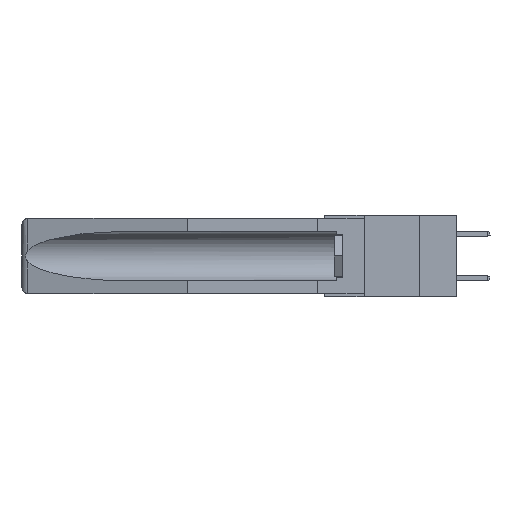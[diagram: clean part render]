
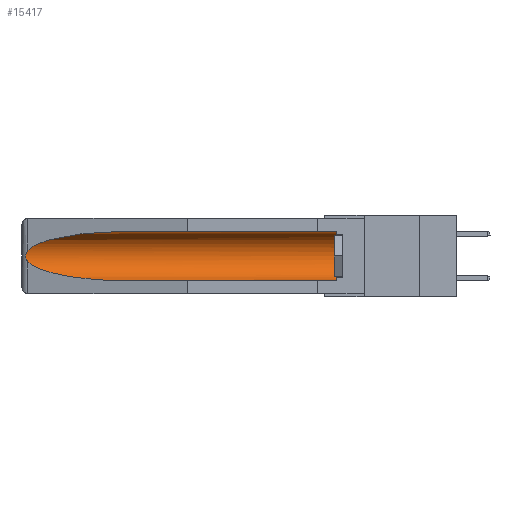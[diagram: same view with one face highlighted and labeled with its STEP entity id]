
A CAD part, left-side view. The second image highlights one B-rep face of the part: STEP entity #15417.
In plain terms, the highlighted cylindrical face has radius 2.857 mm (diameter 5.715 mm), a partial arc.
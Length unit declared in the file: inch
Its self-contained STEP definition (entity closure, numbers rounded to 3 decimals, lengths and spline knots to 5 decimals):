
#425 = CYLINDRICAL_SURFACE ( 'NONE', #18403, 0.1125 ) ;
#969 = ORIENTED_EDGE ( 'NONE', *, *, #23321, .T. ) ;
#1375 = CARTESIAN_POINT ( 'NONE',  ( 0.155, 1.07973, -0.059 ) ) ;
#1829 = CARTESIAN_POINT ( 'NONE',  ( 0.2675, 1.53308, -0.17534 ) ) ;
#2647 = CARTESIAN_POINT ( 'NONE',  ( 0.155, -0.30754, -0.284 ) ) ;
#3432 = DIRECTION ( 'NONE',  ( 0., -1., 0. ) ) ;
#3469 = CARTESIAN_POINT ( 'NONE',  ( 0.155, 1.07973, -0.059 ) ) ;
#3788 = CARTESIAN_POINT ( 'NONE',  ( 0.21114, 1.30732, -0.284 ) ) ;
#3941 = FACE_OUTER_BOUND ( 'NONE', #4573, .T. ) ;
#4108 = ORIENTED_EDGE ( 'NONE', *, *, #27617, .T. ) ;
#4573 = EDGE_LOOP ( 'NONE', ( #5721, #26102, #969, #15722, #8129, #4108 ) ) ;
#4890 = DIRECTION ( 'NONE',  ( 0., 1., 0. ) ) ;
#5669 = CARTESIAN_POINT ( 'NONE',  ( 0.155, -0.30754, -0.059 ) ) ;
#5721 = ORIENTED_EDGE ( 'NONE', *, *, #13810, .T. ) ;
#6030 = CARTESIAN_POINT ( 'NONE',  ( 0.25451, 1.48313, -0.24835 ) ) ;
#6208 = CARTESIAN_POINT ( 'NONE',  ( 0.2673, 1.5327, -0.16383 ) ) ;
#6499 = CARTESIAN_POINT ( 'NONE',  ( 0.2673, 1.53269, -0.17917 ) ) ;
#6960 = CIRCLE ( 'NONE', #20569, 0.1125 ) ;
#8078 = B_SPLINE_CURVE_WITH_KNOTS ( 'NONE', 3,
 ( #19342, #12297, #22026, #6208, #23766, #1829, #6499, #26342, #15083, #15363 ),
 .UNSPECIFIED., .F., .F.,
 ( 4, 2, 2, 2, 4 ),
 ( 0., 0.00029, 0.00058, 0.00087, 0.00117 ),
 .UNSPECIFIED. ) ;
#8129 = ORIENTED_EDGE ( 'NONE', *, *, #27659, .T. ) ;
#8328 = CARTESIAN_POINT ( 'NONE',  ( 0.155, 1.07973, -0.284 ) ) ;
#8351 = CARTESIAN_POINT ( 'NONE',  ( 0.25451, 1.48313, -0.09465 ) ) ;
#9335 = VERTEX_POINT ( 'NONE', #19766 ) ;
#9618 = DIRECTION ( 'NONE',  ( 0., 0., 1. ) ) ;
#11396 = VERTEX_POINT ( 'NONE', #3469 ) ;
#12297 = CARTESIAN_POINT ( 'NONE',  ( 0.26597, 1.52961, -0.15275 ) ) ;
#13810 = EDGE_CURVE ( 'NONE', #11396, #9335, #17532, .T. ) ;
#14111 = CARTESIAN_POINT ( 'NONE',  ( 0.155, -0.30754, -0.1715 ) ) ;
#15083 = CARTESIAN_POINT ( 'NONE',  ( 0.26597, 1.5296, -0.19026 ) ) ;
#15363 = CARTESIAN_POINT ( 'NONE',  ( 0.26537, 1.52718, -0.19328 ) ) ;
#15389 = VERTEX_POINT ( 'NONE', #16059 ) ;
#15417 = ADVANCED_FACE ( 'NONE', ( #3941 ), #425, .F. ) ;
#15722 = ORIENTED_EDGE ( 'NONE', *, *, #21259, .F. ) ;
#16059 = CARTESIAN_POINT ( 'NONE',  ( 0.155, 0.126, -0.059 ) ) ;
#16081 = CARTESIAN_POINT ( 'NONE',  ( 0.26537, 1.52718, -0.19328 ) ) ;
#16773 = CARTESIAN_POINT ( 'NONE',  ( 0.155, 0.126, -0.1715 ) ) ;
#17495 = CARTESIAN_POINT ( 'NONE',  ( 0.155, 1.07973, -0.284 ) ) ;
#17532 =( BOUNDED_CURVE ( )  B_SPLINE_CURVE ( 3, ( #1375, #21564, #8351, #28022 ),
 .UNSPECIFIED., .F., .F. ) 
 B_SPLINE_CURVE_WITH_KNOTS ( ( 4, 4 ),
 ( 4.71239, 6.08839 ),
 .UNSPECIFIED. ) 
 CURVE ( )  GEOMETRIC_REPRESENTATION_ITEM ( )  RATIONAL_B_SPLINE_CURVE ( ( 1., 0.848, 0.848, 1. ) ) 
 REPRESENTATION_ITEM ( '' )  );
#17902 = VERTEX_POINT ( 'NONE', #17495 ) ;
#18403 = AXIS2_PLACEMENT_3D ( 'NONE', #14111, #27607, #9618 ) ;
#19000 = DIRECTION ( 'NONE',  ( 0., 0., 1. ) ) ;
#19342 = CARTESIAN_POINT ( 'NONE',  ( 0.26537, 1.52718, -0.14972 ) ) ;
#19766 = CARTESIAN_POINT ( 'NONE',  ( 0.26537, 1.52718, -0.14972 ) ) ;
#20569 = AXIS2_PLACEMENT_3D ( 'NONE', #16773, #3432, #19000 ) ;
#20697 = VERTEX_POINT ( 'NONE', #22588 ) ;
#21259 = EDGE_CURVE ( 'NONE', #20697, #17902, #24244, .T. ) ;
#21494 = EDGE_CURVE ( 'NONE', #9335, #22833, #8078, .T. ) ;
#21564 = CARTESIAN_POINT ( 'NONE',  ( 0.21114, 1.30732, -0.059 ) ) ;
#22026 = CARTESIAN_POINT ( 'NONE',  ( 0.26654, 1.53092, -0.15636 ) ) ;
#22588 = CARTESIAN_POINT ( 'NONE',  ( 0.155, 0.126, -0.284 ) ) ;
#22833 = VERTEX_POINT ( 'NONE', #16081 ) ;
#23321 = EDGE_CURVE ( 'NONE', #22833, #17902, #28654, .T. ) ;
#23763 = CARTESIAN_POINT ( 'NONE',  ( 0.26537, 1.52718, -0.19328 ) ) ;
#23766 = CARTESIAN_POINT ( 'NONE',  ( 0.2675, 1.53308, -0.16763 ) ) ;
#24244 = LINE ( 'NONE', #2647, #25297 ) ;
#25297 = VECTOR ( 'NONE', #4890, 39.37008 ) ;
#26102 = ORIENTED_EDGE ( 'NONE', *, *, #21494, .T. ) ;
#26342 = CARTESIAN_POINT ( 'NONE',  ( 0.26655, 1.53094, -0.18657 ) ) ;
#26712 = VECTOR ( 'NONE', #27634, 39.37008 ) ;
#27607 = DIRECTION ( 'NONE',  ( 0., 1., 0. ) ) ;
#27617 = EDGE_CURVE ( 'NONE', #15389, #11396, #28096, .T. ) ;
#27634 = DIRECTION ( 'NONE',  ( 0., 1., 0. ) ) ;
#27659 = EDGE_CURVE ( 'NONE', #20697, #15389, #6960, .T. ) ;
#28022 = CARTESIAN_POINT ( 'NONE',  ( 0.26537, 1.52718, -0.14972 ) ) ;
#28096 = LINE ( 'NONE', #5669, #26712 ) ;
#28654 =( BOUNDED_CURVE ( )  B_SPLINE_CURVE ( 3, ( #23763, #6030, #3788, #8328 ),
 .UNSPECIFIED., .F., .F. ) 
 B_SPLINE_CURVE_WITH_KNOTS ( ( 4, 4 ),
 ( 0.1948, 1.5708 ),
 .UNSPECIFIED. ) 
 CURVE ( )  GEOMETRIC_REPRESENTATION_ITEM ( )  RATIONAL_B_SPLINE_CURVE ( ( 1., 0.848, 0.848, 1. ) ) 
 REPRESENTATION_ITEM ( '' )  );
